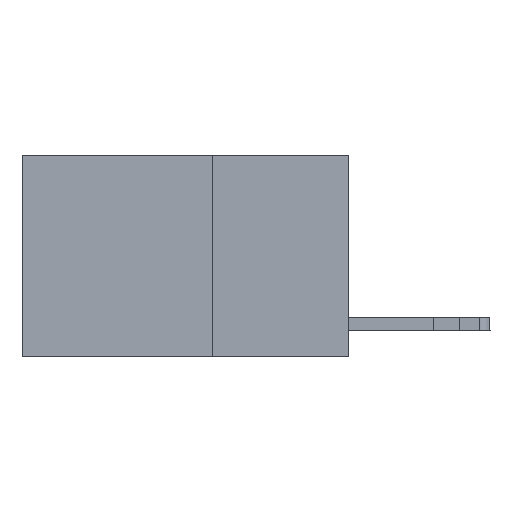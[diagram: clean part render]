
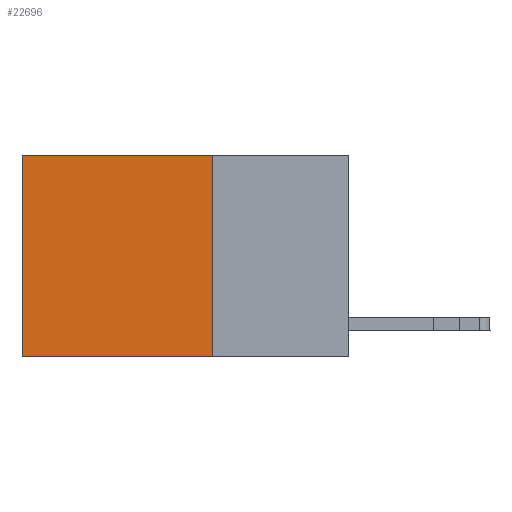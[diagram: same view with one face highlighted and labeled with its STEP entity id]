
A CAD part, left-side view. The second image highlights one B-rep face of the part: STEP entity #22696.
In plain terms, the highlighted planar face has unit normal (-1, 0, 0).
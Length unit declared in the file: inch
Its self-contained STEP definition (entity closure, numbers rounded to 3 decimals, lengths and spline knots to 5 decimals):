
#194 = ORIENTED_EDGE ( 'NONE', *, *, #20270, .F. ) ;
#336 = CARTESIAN_POINT ( 'NONE',  ( 0.2625, 0.25, -0.37 ) ) ;
#613 = CARTESIAN_POINT ( 'NONE',  ( 0.2625, 0.6, 0. ) ) ;
#1650 = DIRECTION ( 'NONE',  ( 0., 1., 0. ) ) ;
#2160 = AXIS2_PLACEMENT_3D ( 'NONE', #22030, #22158, #8849 ) ;
#2773 = VERTEX_POINT ( 'NONE', #10618 ) ;
#3421 = ORIENTED_EDGE ( 'NONE', *, *, #7545, .F. ) ;
#3466 = VECTOR ( 'NONE', #7304, 39.37008 ) ;
#5006 = LINE ( 'NONE', #9109, #19869 ) ;
#6626 = FACE_OUTER_BOUND ( 'NONE', #10577, .T. ) ;
#7304 = DIRECTION ( 'NONE',  ( 0., 1., 0. ) ) ;
#7545 = EDGE_CURVE ( 'NONE', #15171, #12422, #20744, .T. ) ;
#8849 = DIRECTION ( 'NONE',  ( 0., 0., -1. ) ) ;
#9109 = CARTESIAN_POINT ( 'NONE',  ( 0.2625, 0.25, 0. ) ) ;
#9661 = DIRECTION ( 'NONE',  ( 0., 0., -1. ) ) ;
#9855 = ORIENTED_EDGE ( 'NONE', *, *, #17371, .T. ) ;
#10474 = PLANE ( 'NONE',  #2160 ) ;
#10577 = EDGE_LOOP ( 'NONE', ( #24394, #3421, #194, #9855 ) ) ;
#10618 = CARTESIAN_POINT ( 'NONE',  ( 0.2625, 0.25, 0. ) ) ;
#10824 = DIRECTION ( 'NONE',  ( 0., 0., -1. ) ) ;
#11810 = LINE ( 'NONE', #613, #21764 ) ;
#12422 = VERTEX_POINT ( 'NONE', #23708 ) ;
#12976 = LINE ( 'NONE', #18835, #13379 ) ;
#13379 = VECTOR ( 'NONE', #1650, 39.37008 ) ;
#15171 = VERTEX_POINT ( 'NONE', #336 ) ;
#16349 = EDGE_CURVE ( 'NONE', #22318, #12422, #11810, .T. ) ;
#17371 = EDGE_CURVE ( 'NONE', #2773, #22318, #12976, .T. ) ;
#18835 = CARTESIAN_POINT ( 'NONE',  ( 0.2625, 0.25, 0. ) ) ;
#18842 = CARTESIAN_POINT ( 'NONE',  ( 0.2625, 0.25, -0.37 ) ) ;
#19869 = VECTOR ( 'NONE', #10824, 39.37008 ) ;
#20270 = EDGE_CURVE ( 'NONE', #2773, #15171, #5006, .T. ) ;
#20744 = LINE ( 'NONE', #18842, #3466 ) ;
#21764 = VECTOR ( 'NONE', #9661, 39.37008 ) ;
#22030 = CARTESIAN_POINT ( 'NONE',  ( 0.2625, 0.25, 0. ) ) ;
#22158 = DIRECTION ( 'NONE',  ( 1., 0., 0. ) ) ;
#22318 = VERTEX_POINT ( 'NONE', #22481 ) ;
#22481 = CARTESIAN_POINT ( 'NONE',  ( 0.2625, 0.6, 0. ) ) ;
#22696 = ADVANCED_FACE ( 'NONE', ( #6626 ), #10474, .F. ) ;
#23708 = CARTESIAN_POINT ( 'NONE',  ( 0.2625, 0.6, -0.37 ) ) ;
#24394 = ORIENTED_EDGE ( 'NONE', *, *, #16349, .T. ) ;
